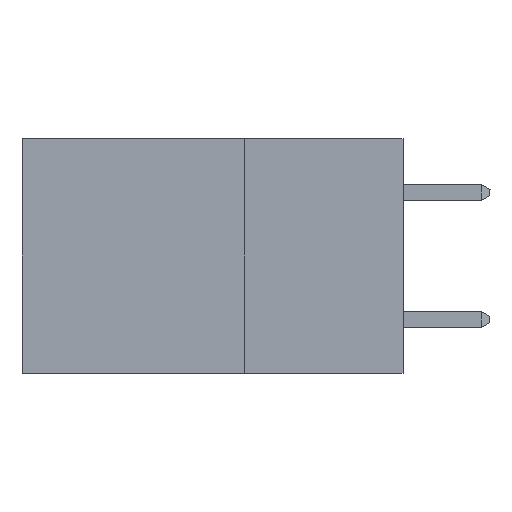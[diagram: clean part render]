
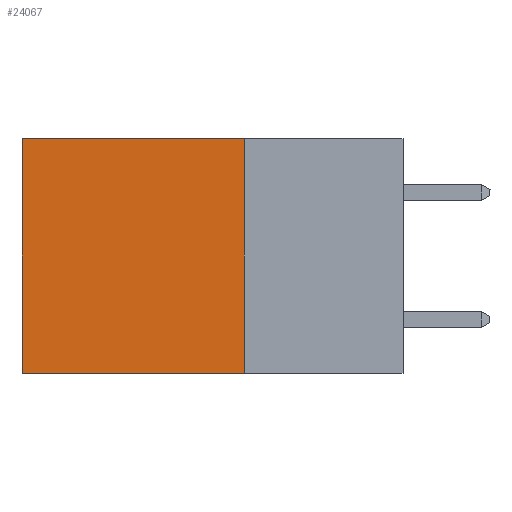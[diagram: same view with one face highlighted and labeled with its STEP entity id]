
A CAD part, left-side view. The second image highlights one B-rep face of the part: STEP entity #24067.
In plain terms, the highlighted planar face has unit normal (-1, 0, 0).
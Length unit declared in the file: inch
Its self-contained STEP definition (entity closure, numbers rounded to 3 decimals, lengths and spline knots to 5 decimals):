
#382 = CARTESIAN_POINT ( 'NONE',  ( 0.2875, 0.25, 0. ) ) ;
#1166 = CARTESIAN_POINT ( 'NONE',  ( 0.2875, 0.25, 0. ) ) ;
#6761 = VERTEX_POINT ( 'NONE', #10682 ) ;
#6804 = ORIENTED_EDGE ( 'NONE', *, *, #35465, .F. ) ;
#7065 = DIRECTION ( 'NONE',  ( 1., 0., 0. ) ) ;
#7243 = CARTESIAN_POINT ( 'NONE',  ( 0.2875, 0.6, 0. ) ) ;
#8690 = VERTEX_POINT ( 'NONE', #33151 ) ;
#10682 = CARTESIAN_POINT ( 'NONE',  ( 0.2875, 0.25, 0. ) ) ;
#10992 = EDGE_CURVE ( 'NONE', #6761, #8690, #30667, .T. ) ;
#11486 = DIRECTION ( 'NONE',  ( 0., 1., 0. ) ) ;
#11542 = AXIS2_PLACEMENT_3D ( 'NONE', #382, #7065, #20608 ) ;
#11978 = VECTOR ( 'NONE', #14994, 39.37008 ) ;
#14111 = DIRECTION ( 'NONE',  ( 0., 0., -1. ) ) ;
#14884 = LINE ( 'NONE', #37696, #30078 ) ;
#14994 = DIRECTION ( 'NONE',  ( 0., 1., 0. ) ) ;
#17797 = VECTOR ( 'NONE', #11486, 39.37008 ) ;
#18166 = EDGE_LOOP ( 'NONE', ( #27737, #6804, #31435, #38560 ) ) ;
#19723 = LINE ( 'NONE', #7243, #33804 ) ;
#20608 = DIRECTION ( 'NONE',  ( 0., 0., -1. ) ) ;
#21491 = CARTESIAN_POINT ( 'NONE',  ( 0.2875, 0.25, -0.37 ) ) ;
#22358 = CARTESIAN_POINT ( 'NONE',  ( 0.2875, 0.25, -0.37 ) ) ;
#23349 = EDGE_CURVE ( 'NONE', #6761, #26164, #14884, .T. ) ;
#24067 = ADVANCED_FACE ( 'NONE', ( #30081 ), #39973, .F. ) ;
#25481 = VERTEX_POINT ( 'NONE', #27094 ) ;
#26164 = VERTEX_POINT ( 'NONE', #22358 ) ;
#27094 = CARTESIAN_POINT ( 'NONE',  ( 0.2875, 0.6, -0.37 ) ) ;
#27737 = ORIENTED_EDGE ( 'NONE', *, *, #31161, .T. ) ;
#30078 = VECTOR ( 'NONE', #31053, 39.37008 ) ;
#30081 = FACE_OUTER_BOUND ( 'NONE', #18166, .T. ) ;
#30667 = LINE ( 'NONE', #1166, #17797 ) ;
#31053 = DIRECTION ( 'NONE',  ( 0., 0., -1. ) ) ;
#31161 = EDGE_CURVE ( 'NONE', #8690, #25481, #19723, .T. ) ;
#31435 = ORIENTED_EDGE ( 'NONE', *, *, #23349, .F. ) ;
#33151 = CARTESIAN_POINT ( 'NONE',  ( 0.2875, 0.6, 0. ) ) ;
#33804 = VECTOR ( 'NONE', #14111, 39.37008 ) ;
#34614 = LINE ( 'NONE', #21491, #11978 ) ;
#35465 = EDGE_CURVE ( 'NONE', #26164, #25481, #34614, .T. ) ;
#37696 = CARTESIAN_POINT ( 'NONE',  ( 0.2875, 0.25, 0. ) ) ;
#38560 = ORIENTED_EDGE ( 'NONE', *, *, #10992, .T. ) ;
#39973 = PLANE ( 'NONE',  #11542 ) ;
